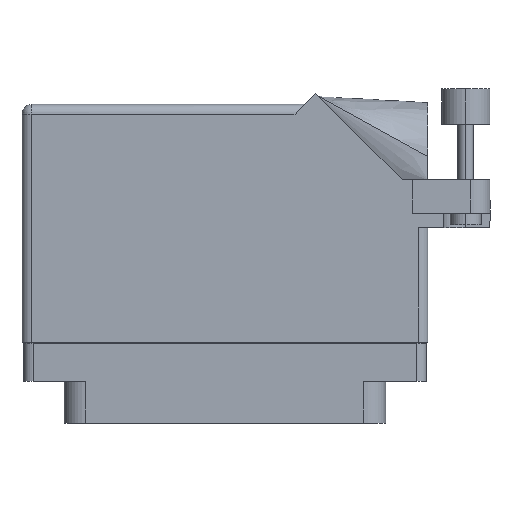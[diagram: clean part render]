
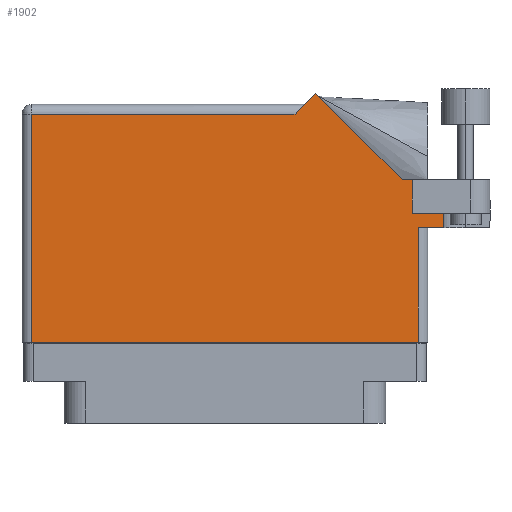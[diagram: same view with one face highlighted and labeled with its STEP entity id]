
A CAD part, front view. The second image highlights one B-rep face of the part: STEP entity #1902.
In plain terms, the highlighted face is planar.
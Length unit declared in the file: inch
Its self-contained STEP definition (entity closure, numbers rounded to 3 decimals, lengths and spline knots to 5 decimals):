
#281 = EDGE_CURVE ( 'NONE', #14213, #25402, #10987, .T. ) ;
#421 = ORIENTED_EDGE ( 'NONE', *, *, #12193, .T. ) ;
#1087 = CARTESIAN_POINT ( 'NONE',  ( 1.306, 0.637, 0.455 ) ) ;
#1489 = VERTEX_POINT ( 'NONE', #4751 ) ;
#1867 = CARTESIAN_POINT ( 'NONE',  ( 1.14042, 0.944, 0.455 ) ) ;
#1872 = CARTESIAN_POINT ( 'NONE',  ( 1.244, -0.1, 0.455 ) ) ;
#1902 = ADVANCED_FACE ( 'NONE', ( #3839 ), #14559, .F. ) ;
#2613 = VECTOR ( 'NONE', #45254, 39.37008 ) ;
#2788 = VECTOR ( 'NONE', #3396, 39.37008 ) ;
#3396 = DIRECTION ( 'NONE',  ( 0., -1., 0. ) ) ;
#3723 = EDGE_CURVE ( 'NONE', #4464, #11332, #20358, .T. ) ;
#3839 = FACE_OUTER_BOUND ( 'NONE', #6326, .T. ) ;
#4464 = VERTEX_POINT ( 'NONE', #44135 ) ;
#4751 = CARTESIAN_POINT ( 'NONE',  ( 0.451, 1.368, 0.455 ) ) ;
#4833 = LINE ( 'NONE', #27266, #32138 ) ;
#5198 = EDGE_CURVE ( 'NONE', #15955, #22374, #34041, .T. ) ;
#6326 = EDGE_LOOP ( 'NONE', ( #49626, #40006, #15303, #22378, #25604, #44338, #39413, #27256, #7968, #421, #7039 ) ) ;
#6462 = LINE ( 'NONE', #29163, #50613 ) ;
#6825 = CARTESIAN_POINT ( 'NONE',  ( -1.306, -0.1, 0.455 ) ) ;
#6931 = CARTESIAN_POINT ( 'NONE',  ( 1.4075, 1.06177, 0.455 ) ) ;
#7039 = ORIENTED_EDGE ( 'NONE', *, *, #33321, .T. ) ;
#7329 = CARTESIAN_POINT ( 'NONE',  ( -1.244, -0.1, 0.455 ) ) ;
#7801 = CARTESIAN_POINT ( 'NONE',  ( 1.244, 0.637, 0.455 ) ) ;
#7872 = LINE ( 'NONE', #6825, #50749 ) ;
#7968 = ORIENTED_EDGE ( 'NONE', *, *, #51047, .T. ) ;
#9434 = VERTEX_POINT ( 'NONE', #7329 ) ;
#10987 = LINE ( 'NONE', #6931, #2788 ) ;
#11332 = VERTEX_POINT ( 'NONE', #50807 ) ;
#12193 = EDGE_CURVE ( 'NONE', #1489, #24718, #6462, .T. ) ;
#12593 = VECTOR ( 'NONE', #20188, 39.37008 ) ;
#13428 = VECTOR ( 'NONE', #19502, 39.37008 ) ;
#14213 = VERTEX_POINT ( 'NONE', #22955 ) ;
#14559 = PLANE ( 'NONE',  #47326 ) ;
#14620 = LINE ( 'NONE', #39546, #24707 ) ;
#15303 = ORIENTED_EDGE ( 'NONE', *, *, #44128, .T. ) ;
#15955 = VERTEX_POINT ( 'NONE', #1867 ) ;
#16523 = VECTOR ( 'NONE', #49662, 39.37008 ) ;
#17416 = CARTESIAN_POINT ( 'NONE',  ( 1.706, 0.944, 0.455 ) ) ;
#17721 = DIRECTION ( 'NONE',  ( -1., 0., 0. ) ) ;
#19502 = DIRECTION ( 'NONE',  ( 0., 1., 0. ) ) ;
#19788 = EDGE_CURVE ( 'NONE', #9434, #38191, #7872, .T. ) ;
#20188 = DIRECTION ( 'NONE',  ( -0.707, 0.707, 0. ) ) ;
#20358 = LINE ( 'NONE', #39765, #13428 ) ;
#22374 = VERTEX_POINT ( 'NONE', #30722 ) ;
#22378 = ORIENTED_EDGE ( 'NONE', *, *, #281, .F. ) ;
#22955 = CARTESIAN_POINT ( 'NONE',  ( 1.4075, 0.731, 0.455 ) ) ;
#23126 = VECTOR ( 'NONE', #48270, 39.37008 ) ;
#23377 = DIRECTION ( 'NONE',  ( 0., 0., -1. ) ) ;
#24707 = VECTOR ( 'NONE', #31118, 39.37008 ) ;
#24718 = VERTEX_POINT ( 'NONE', #46395 ) ;
#25402 = VERTEX_POINT ( 'NONE', #48464 ) ;
#25604 = ORIENTED_EDGE ( 'NONE', *, *, #41644, .F. ) ;
#27242 = LINE ( 'NONE', #17416, #16523 ) ;
#27256 = ORIENTED_EDGE ( 'NONE', *, *, #5198, .T. ) ;
#27266 = CARTESIAN_POINT ( 'NONE',  ( 1.206, 0.731, 0.455 ) ) ;
#27995 = EDGE_CURVE ( 'NONE', #38191, #39073, #49554, .T. ) ;
#28335 = LINE ( 'NONE', #51378, #45953 ) ;
#28482 = DIRECTION ( 'NONE',  ( 1., 0., 0. ) ) ;
#29163 = CARTESIAN_POINT ( 'NONE',  ( -1.306, 1.368, 0.455 ) ) ;
#29960 = EDGE_CURVE ( 'NONE', #11332, #15955, #27242, .T. ) ;
#30722 = CARTESIAN_POINT ( 'NONE',  ( 0.58371, 1.50071, 0.455 ) ) ;
#31118 = DIRECTION ( 'NONE',  ( 0., -1., 0. ) ) ;
#31320 = DIRECTION ( 'NONE',  ( 1., 0., 0. ) ) ;
#31794 = CARTESIAN_POINT ( 'NONE',  ( 1.244, 0.637, 0.455 ) ) ;
#32138 = VECTOR ( 'NONE', #31320, 39.37008 ) ;
#33321 = EDGE_CURVE ( 'NONE', #24718, #9434, #14620, .T. ) ;
#34041 = LINE ( 'NONE', #40955, #12593 ) ;
#35533 = CARTESIAN_POINT ( 'NONE',  ( -1.306, 1.43, 0.455 ) ) ;
#38191 = VERTEX_POINT ( 'NONE', #1872 ) ;
#39073 = VERTEX_POINT ( 'NONE', #31794 ) ;
#39413 = ORIENTED_EDGE ( 'NONE', *, *, #29960, .T. ) ;
#39546 = CARTESIAN_POINT ( 'NONE',  ( -1.244, -0.1, 0.455 ) ) ;
#39765 = CARTESIAN_POINT ( 'NONE',  ( 1.206, 0.731, 0.455 ) ) ;
#40006 = ORIENTED_EDGE ( 'NONE', *, *, #27995, .T. ) ;
#40955 = CARTESIAN_POINT ( 'NONE',  ( 1.14042, 0.944, 0.455 ) ) ;
#41644 = EDGE_CURVE ( 'NONE', #4464, #14213, #4833, .T. ) ;
#42732 = DIRECTION ( 'NONE',  ( -1., 0., 0. ) ) ;
#44128 = EDGE_CURVE ( 'NONE', #39073, #25402, #50543, .T. ) ;
#44135 = CARTESIAN_POINT ( 'NONE',  ( 1.206, 0.731, 0.455 ) ) ;
#44338 = ORIENTED_EDGE ( 'NONE', *, *, #3723, .T. ) ;
#45254 = DIRECTION ( 'NONE',  ( 1., 0., 0. ) ) ;
#45953 = VECTOR ( 'NONE', #52116, 39.37008 ) ;
#46395 = CARTESIAN_POINT ( 'NONE',  ( -1.244, 1.368, 0.455 ) ) ;
#47326 = AXIS2_PLACEMENT_3D ( 'NONE', #35533, #23377, #42732 ) ;
#48270 = DIRECTION ( 'NONE',  ( 0., 1., 0. ) ) ;
#48464 = CARTESIAN_POINT ( 'NONE',  ( 1.4075, 0.637, 0.455 ) ) ;
#49554 = LINE ( 'NONE', #7801, #23126 ) ;
#49626 = ORIENTED_EDGE ( 'NONE', *, *, #19788, .T. ) ;
#49662 = DIRECTION ( 'NONE',  ( -1., 0., 0. ) ) ;
#50543 = LINE ( 'NONE', #1087, #2613 ) ;
#50613 = VECTOR ( 'NONE', #17721, 39.37008 ) ;
#50749 = VECTOR ( 'NONE', #28482, 39.37008 ) ;
#50807 = CARTESIAN_POINT ( 'NONE',  ( 1.206, 0.944, 0.455 ) ) ;
#51047 = EDGE_CURVE ( 'NONE', #22374, #1489, #28335, .T. ) ;
#51378 = CARTESIAN_POINT ( 'NONE',  ( 0.513, 1.43, 0.455 ) ) ;
#52116 = DIRECTION ( 'NONE',  ( -0.707, -0.707, 0. ) ) ;
